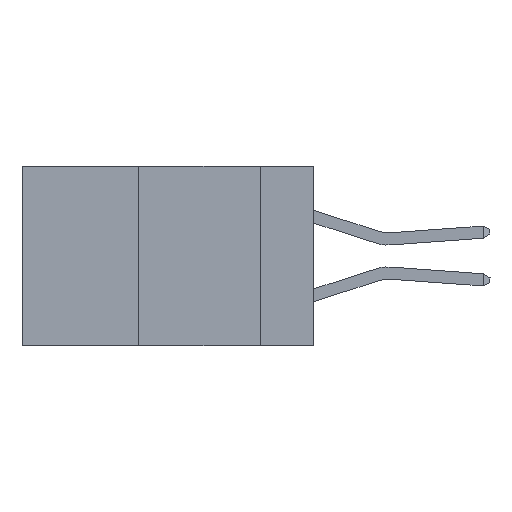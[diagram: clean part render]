
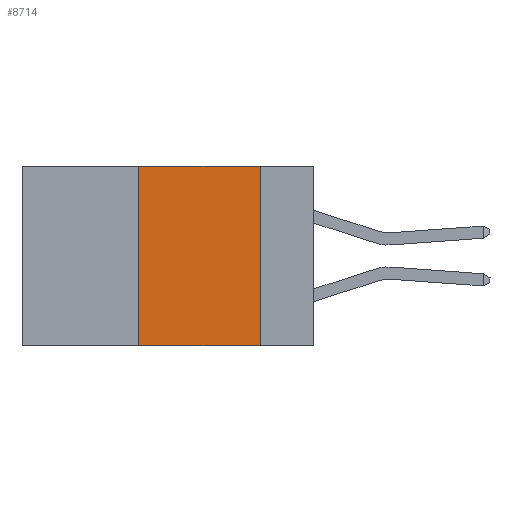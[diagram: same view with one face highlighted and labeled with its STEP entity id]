
A CAD part, left-side view. The second image highlights one B-rep face of the part: STEP entity #8714.
In plain terms, the highlighted planar face has unit normal (-1, 0, 0).
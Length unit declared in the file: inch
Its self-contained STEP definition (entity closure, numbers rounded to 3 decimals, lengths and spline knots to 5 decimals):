
#69 = EDGE_CURVE ( 'NONE', #4684, #11857, #10958, .T. ) ;
#1296 = VECTOR ( 'NONE', #7270, 39.37008 ) ;
#1527 = CARTESIAN_POINT ( 'NONE',  ( 0., 0.11, 0. ) ) ;
#1581 = CARTESIAN_POINT ( 'NONE',  ( 0., 0.11, -0.37 ) ) ;
#1659 = CARTESIAN_POINT ( 'NONE',  ( 0., 0.36, 0. ) ) ;
#1729 = EDGE_LOOP ( 'NONE', ( #2917, #6650, #10886, #5989 ) ) ;
#2329 = VECTOR ( 'NONE', #12170, 39.37008 ) ;
#2575 = CARTESIAN_POINT ( 'NONE',  ( 0., 0.6, 0. ) ) ;
#2808 = CARTESIAN_POINT ( 'NONE',  ( 0., 0.36, -0.37 ) ) ;
#2917 = ORIENTED_EDGE ( 'NONE', *, *, #11416, .F. ) ;
#3215 = VERTEX_POINT ( 'NONE', #2808 ) ;
#3419 = PLANE ( 'NONE',  #6729 ) ;
#3550 = CARTESIAN_POINT ( 'NONE',  ( 0., 0.11, 0. ) ) ;
#3776 = VECTOR ( 'NONE', #11194, 39.37008 ) ;
#4684 = VERTEX_POINT ( 'NONE', #5661 ) ;
#5661 = CARTESIAN_POINT ( 'NONE',  ( 0., 0.36, 0. ) ) ;
#5989 = ORIENTED_EDGE ( 'NONE', *, *, #7086, .T. ) ;
#6293 = DIRECTION ( 'NONE',  ( 1., 0., 0. ) ) ;
#6650 = ORIENTED_EDGE ( 'NONE', *, *, #69, .F. ) ;
#6729 = AXIS2_PLACEMENT_3D ( 'NONE', #2575, #6293, #8203 ) ;
#7086 = EDGE_CURVE ( 'NONE', #3215, #8219, #11434, .T. ) ;
#7270 = DIRECTION ( 'NONE',  ( 0., 0., -1. ) ) ;
#7987 = EDGE_CURVE ( 'NONE', #3215, #4684, #11817, .T. ) ;
#8203 = DIRECTION ( 'NONE',  ( 0., 0., -1. ) ) ;
#8219 = VERTEX_POINT ( 'NONE', #1581 ) ;
#8318 = DIRECTION ( 'NONE',  ( 0., 0., 1. ) ) ;
#8714 = ADVANCED_FACE ( 'NONE', ( #12155 ), #3419, .F. ) ;
#8930 = LINE ( 'NONE', #3550, #1296 ) ;
#10231 = VECTOR ( 'NONE', #8318, 39.37008 ) ;
#10263 = CARTESIAN_POINT ( 'NONE',  ( 0., 0.6, -0.37 ) ) ;
#10288 = CARTESIAN_POINT ( 'NONE',  ( 0., 0.6, 0. ) ) ;
#10886 = ORIENTED_EDGE ( 'NONE', *, *, #7987, .F. ) ;
#10958 = LINE ( 'NONE', #10288, #3776 ) ;
#11194 = DIRECTION ( 'NONE',  ( 0., -1., 0. ) ) ;
#11416 = EDGE_CURVE ( 'NONE', #11857, #8219, #8930, .T. ) ;
#11434 = LINE ( 'NONE', #10263, #2329 ) ;
#11817 = LINE ( 'NONE', #1659, #10231 ) ;
#11857 = VERTEX_POINT ( 'NONE', #1527 ) ;
#12155 = FACE_OUTER_BOUND ( 'NONE', #1729, .T. ) ;
#12170 = DIRECTION ( 'NONE',  ( 0., -1., 0. ) ) ;
